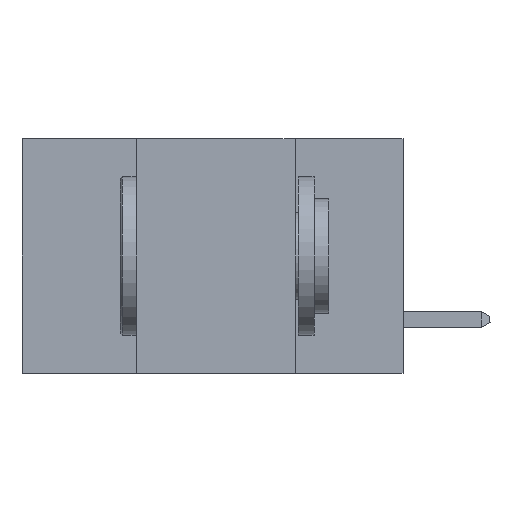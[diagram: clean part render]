
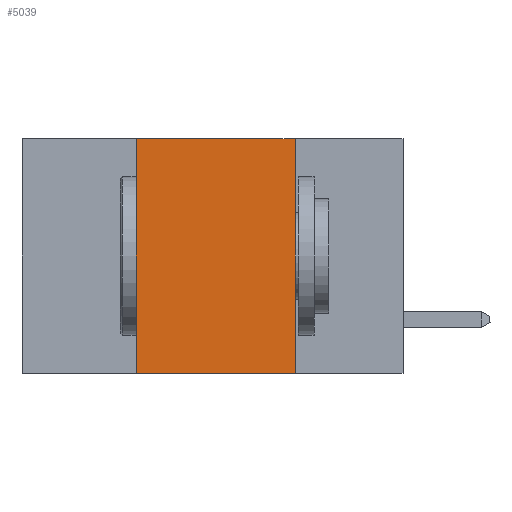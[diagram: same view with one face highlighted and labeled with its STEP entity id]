
A CAD part, left-side view. The second image highlights one B-rep face of the part: STEP entity #5039.
In plain terms, the highlighted planar face has unit normal (-1, 0, 0).
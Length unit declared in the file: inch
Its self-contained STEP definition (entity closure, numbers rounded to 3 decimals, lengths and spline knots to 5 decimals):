
#1338 = ORIENTED_EDGE ( 'NONE', *, *, #6747, .T. ) ;
#1649 = CARTESIAN_POINT ( 'NONE',  ( 0., 0.42, 0. ) ) ;
#2043 = VECTOR ( 'NONE', #22357, 39.37008 ) ;
#5039 = ADVANCED_FACE ( 'NONE', ( #22757 ), #21620, .F. ) ;
#6055 = VECTOR ( 'NONE', #29506, 39.37008 ) ;
#6075 = VECTOR ( 'NONE', #16036, 39.37008 ) ;
#6747 = EDGE_CURVE ( 'NONE', #13234, #24444, #11788, .T. ) ;
#6868 = CARTESIAN_POINT ( 'NONE',  ( 0., 0.6, 0. ) ) ;
#7866 = CARTESIAN_POINT ( 'NONE',  ( 0., 0.42, 0. ) ) ;
#8344 = LINE ( 'NONE', #7866, #6055 ) ;
#9628 = CARTESIAN_POINT ( 'NONE',  ( 0., 0.6, 0. ) ) ;
#11788 = LINE ( 'NONE', #19973, #2043 ) ;
#12064 = DIRECTION ( 'NONE',  ( 0., 0., -1. ) ) ;
#13234 = VERTEX_POINT ( 'NONE', #26885 ) ;
#13761 = ORIENTED_EDGE ( 'NONE', *, *, #27252, .F. ) ;
#14357 = ORIENTED_EDGE ( 'NONE', *, *, #27627, .F. ) ;
#14686 = LINE ( 'NONE', #6868, #26755 ) ;
#14843 = CARTESIAN_POINT ( 'NONE',  ( 0., 0.17, -0.37 ) ) ;
#16036 = DIRECTION ( 'NONE',  ( 0., 0., -1. ) ) ;
#18554 = EDGE_CURVE ( 'NONE', #23104, #24444, #24541, .T. ) ;
#18986 = DIRECTION ( 'NONE',  ( 0., -1., 0. ) ) ;
#19973 = CARTESIAN_POINT ( 'NONE',  ( 0., 0.6, -0.37 ) ) ;
#20697 = EDGE_LOOP ( 'NONE', ( #29775, #14357, #13761, #1338 ) ) ;
#21620 = PLANE ( 'NONE',  #28591 ) ;
#22357 = DIRECTION ( 'NONE',  ( 0., -1., 0. ) ) ;
#22757 = FACE_OUTER_BOUND ( 'NONE', #20697, .T. ) ;
#23104 = VERTEX_POINT ( 'NONE', #25218 ) ;
#24444 = VERTEX_POINT ( 'NONE', #14843 ) ;
#24541 = LINE ( 'NONE', #30372, #6075 ) ;
#25218 = CARTESIAN_POINT ( 'NONE',  ( 0., 0.17, 0. ) ) ;
#26470 = DIRECTION ( 'NONE',  ( 1., 0., 0. ) ) ;
#26755 = VECTOR ( 'NONE', #18986, 39.37008 ) ;
#26885 = CARTESIAN_POINT ( 'NONE',  ( 0., 0.42, -0.37 ) ) ;
#27252 = EDGE_CURVE ( 'NONE', #13234, #28151, #8344, .T. ) ;
#27627 = EDGE_CURVE ( 'NONE', #28151, #23104, #14686, .T. ) ;
#28151 = VERTEX_POINT ( 'NONE', #1649 ) ;
#28591 = AXIS2_PLACEMENT_3D ( 'NONE', #9628, #26470, #12064 ) ;
#29506 = DIRECTION ( 'NONE',  ( 0., 0., 1. ) ) ;
#29775 = ORIENTED_EDGE ( 'NONE', *, *, #18554, .F. ) ;
#30372 = CARTESIAN_POINT ( 'NONE',  ( 0., 0.17, 0. ) ) ;
